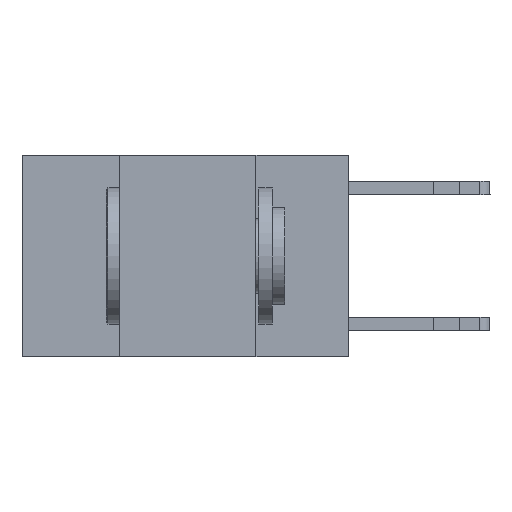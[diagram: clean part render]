
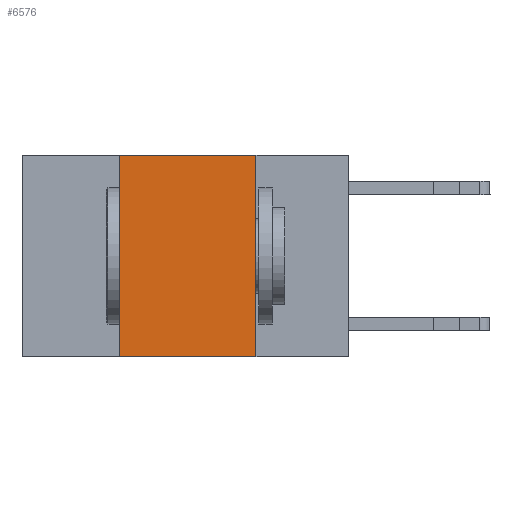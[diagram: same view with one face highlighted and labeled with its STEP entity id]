
A CAD part, left-side view. The second image highlights one B-rep face of the part: STEP entity #6576.
In plain terms, the highlighted planar face has unit normal (-1, 0, 0).
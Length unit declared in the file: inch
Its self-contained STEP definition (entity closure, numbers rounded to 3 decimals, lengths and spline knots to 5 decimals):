
#259 = CARTESIAN_POINT ( 'NONE',  ( 0., 0.42, 0. ) ) ;
#1453 = CARTESIAN_POINT ( 'NONE',  ( 0., 0.6, -0.37 ) ) ;
#2643 = VECTOR ( 'NONE', #18426, 39.37008 ) ;
#2775 = LINE ( 'NONE', #18778, #2643 ) ;
#2850 = VECTOR ( 'NONE', #5178, 39.37008 ) ;
#2922 = LINE ( 'NONE', #5052, #2850 ) ;
#4628 = CARTESIAN_POINT ( 'NONE',  ( 0., 0.42, -0.37 ) ) ;
#5052 = CARTESIAN_POINT ( 'NONE',  ( 0., 0.6, 0. ) ) ;
#5084 = EDGE_CURVE ( 'NONE', #11032, #12355, #2922, .T. ) ;
#5178 = DIRECTION ( 'NONE',  ( 0., -1., 0. ) ) ;
#6576 = ADVANCED_FACE ( 'NONE', ( #17243 ), #8593, .F. ) ;
#8348 = DIRECTION ( 'NONE',  ( 0., 0., -1. ) ) ;
#8370 = DIRECTION ( 'NONE',  ( 1., 0., 0. ) ) ;
#8593 = PLANE ( 'NONE',  #12676 ) ;
#8611 = CARTESIAN_POINT ( 'NONE',  ( 0., 0.6, 0. ) ) ;
#9803 = VECTOR ( 'NONE', #18261, 39.37008 ) ;
#9823 = LINE ( 'NONE', #1453, #9803 ) ;
#11032 = VERTEX_POINT ( 'NONE', #11097 ) ;
#11097 = CARTESIAN_POINT ( 'NONE',  ( 0., 0.42, 0. ) ) ;
#11746 = VERTEX_POINT ( 'NONE', #4628 ) ;
#11996 = EDGE_CURVE ( 'NONE', #11746, #11032, #20719, .T. ) ;
#12355 = VERTEX_POINT ( 'NONE', #19607 ) ;
#12676 = AXIS2_PLACEMENT_3D ( 'NONE', #8611, #8370, #8348 ) ;
#13944 = ORIENTED_EDGE ( 'NONE', *, *, #15341, .F. ) ;
#13961 = ORIENTED_EDGE ( 'NONE', *, *, #5084, .F. ) ;
#14132 = ORIENTED_EDGE ( 'NONE', *, *, #11996, .F. ) ;
#14149 = ORIENTED_EDGE ( 'NONE', *, *, #19028, .T. ) ;
#15341 = EDGE_CURVE ( 'NONE', #12355, #17068, #2775, .T. ) ;
#17068 = VERTEX_POINT ( 'NONE', #19385 ) ;
#17243 = FACE_OUTER_BOUND ( 'NONE', #19824, .T. ) ;
#18261 = DIRECTION ( 'NONE',  ( 0., -1., 0. ) ) ;
#18426 = DIRECTION ( 'NONE',  ( 0., 0., -1. ) ) ;
#18778 = CARTESIAN_POINT ( 'NONE',  ( 0., 0.17, 0. ) ) ;
#19028 = EDGE_CURVE ( 'NONE', #11746, #17068, #9823, .T. ) ;
#19385 = CARTESIAN_POINT ( 'NONE',  ( 0., 0.17, -0.37 ) ) ;
#19607 = CARTESIAN_POINT ( 'NONE',  ( 0., 0.17, 0. ) ) ;
#19824 = EDGE_LOOP ( 'NONE', ( #13944, #13961, #14132, #14149 ) ) ;
#20514 = VECTOR ( 'NONE', #20536, 39.37008 ) ;
#20536 = DIRECTION ( 'NONE',  ( 0., 0., 1. ) ) ;
#20719 = LINE ( 'NONE', #259, #20514 ) ;
